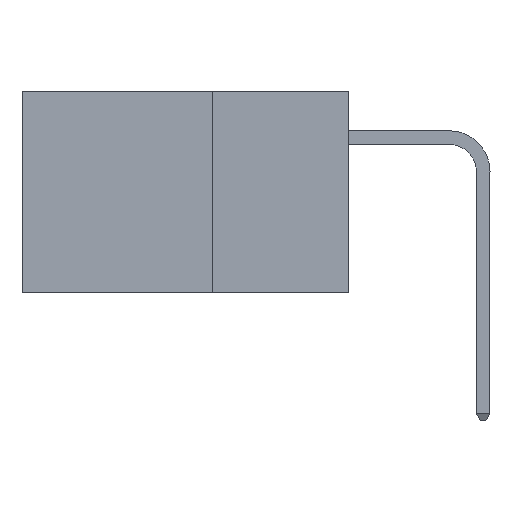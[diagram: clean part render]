
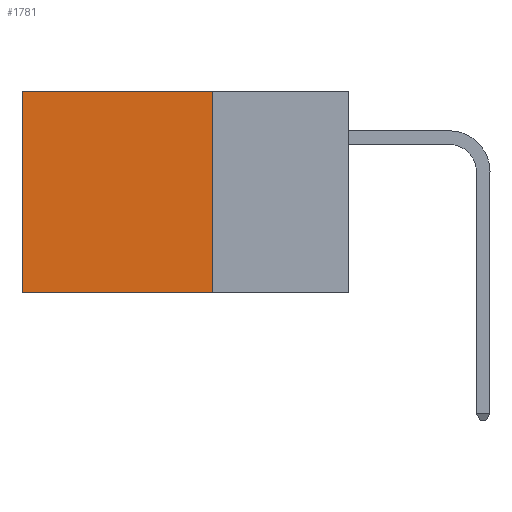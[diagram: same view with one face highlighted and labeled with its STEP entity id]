
A CAD part, left-side view. The second image highlights one B-rep face of the part: STEP entity #1781.
In plain terms, the highlighted planar face has unit normal (-1, 0, 0).
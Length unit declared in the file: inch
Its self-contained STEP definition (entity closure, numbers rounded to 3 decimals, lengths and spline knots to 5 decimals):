
#337 = CARTESIAN_POINT ( 'NONE',  ( 0.2875, 0.6, 0. ) ) ;
#1057 = CARTESIAN_POINT ( 'NONE',  ( 0.2875, 0.25, 0. ) ) ;
#1073 = ORIENTED_EDGE ( 'NONE', *, *, #5251, .F. ) ;
#1253 = CARTESIAN_POINT ( 'NONE',  ( 0.2875, 0.6, -0.37 ) ) ;
#1328 = VERTEX_POINT ( 'NONE', #8804 ) ;
#1781 = ADVANCED_FACE ( 'NONE', ( #1996 ), #7873, .F. ) ;
#1946 = VERTEX_POINT ( 'NONE', #10636 ) ;
#1996 = FACE_OUTER_BOUND ( 'NONE', #7173, .T. ) ;
#2185 = CARTESIAN_POINT ( 'NONE',  ( 0.2875, 0.25, -0.37 ) ) ;
#2649 = DIRECTION ( 'NONE',  ( 0., 1., 0. ) ) ;
#3101 = CARTESIAN_POINT ( 'NONE',  ( 0.2875, 0.25, 0. ) ) ;
#3648 = CARTESIAN_POINT ( 'NONE',  ( 0.2875, 0.25, 0. ) ) ;
#4076 = DIRECTION ( 'NONE',  ( 1., 0., 0. ) ) ;
#4083 = EDGE_CURVE ( 'NONE', #1328, #6713, #5259, .T. ) ;
#5251 = EDGE_CURVE ( 'NONE', #1946, #1328, #11866, .T. ) ;
#5259 = LINE ( 'NONE', #2185, #7486 ) ;
#5852 = ORIENTED_EDGE ( 'NONE', *, *, #8996, .T. ) ;
#6240 = AXIS2_PLACEMENT_3D ( 'NONE', #3101, #4076, #8013 ) ;
#6462 = CARTESIAN_POINT ( 'NONE',  ( 0.2875, 0.6, 0. ) ) ;
#6469 = VECTOR ( 'NONE', #2649, 39.37008 ) ;
#6713 = VERTEX_POINT ( 'NONE', #1253 ) ;
#7173 = EDGE_LOOP ( 'NONE', ( #8489, #11844, #1073, #5852 ) ) ;
#7486 = VECTOR ( 'NONE', #9897, 39.37008 ) ;
#7619 = DIRECTION ( 'NONE',  ( 0., 0., -1. ) ) ;
#7873 = PLANE ( 'NONE',  #6240 ) ;
#8013 = DIRECTION ( 'NONE',  ( 0., 0., -1. ) ) ;
#8489 = ORIENTED_EDGE ( 'NONE', *, *, #10090, .T. ) ;
#8672 = DIRECTION ( 'NONE',  ( 0., 0., -1. ) ) ;
#8804 = CARTESIAN_POINT ( 'NONE',  ( 0.2875, 0.25, -0.37 ) ) ;
#8996 = EDGE_CURVE ( 'NONE', #1946, #9772, #9339, .T. ) ;
#9140 = LINE ( 'NONE', #6462, #12181 ) ;
#9339 = LINE ( 'NONE', #3648, #6469 ) ;
#9772 = VERTEX_POINT ( 'NONE', #337 ) ;
#9897 = DIRECTION ( 'NONE',  ( 0., 1., 0. ) ) ;
#10090 = EDGE_CURVE ( 'NONE', #9772, #6713, #9140, .T. ) ;
#10636 = CARTESIAN_POINT ( 'NONE',  ( 0.2875, 0.25, 0. ) ) ;
#10662 = VECTOR ( 'NONE', #8672, 39.37008 ) ;
#11844 = ORIENTED_EDGE ( 'NONE', *, *, #4083, .F. ) ;
#11866 = LINE ( 'NONE', #1057, #10662 ) ;
#12181 = VECTOR ( 'NONE', #7619, 39.37008 ) ;
